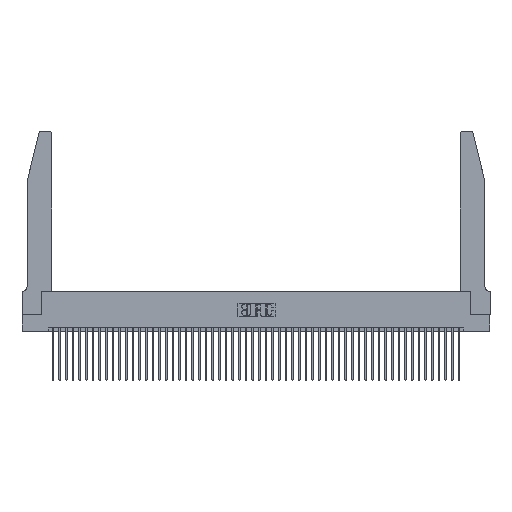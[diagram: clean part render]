
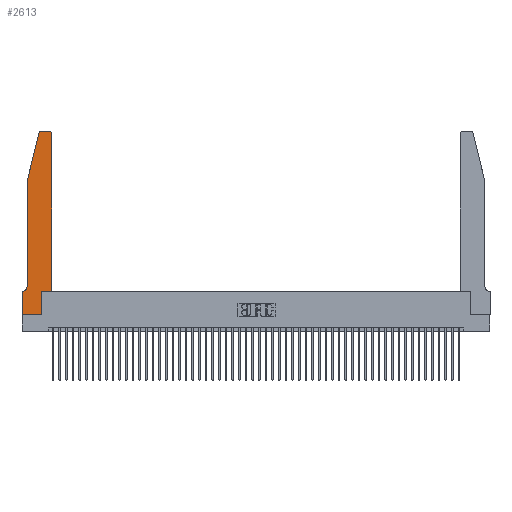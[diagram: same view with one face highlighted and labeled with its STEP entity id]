
A CAD part, top view. The second image highlights one B-rep face of the part: STEP entity #2613.
In plain terms, the highlighted planar face has unit normal (0, 0, 1).
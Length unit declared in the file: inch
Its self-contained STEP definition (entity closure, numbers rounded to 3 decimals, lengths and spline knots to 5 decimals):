
#404 = ORIENTED_EDGE ( 'NONE', *, *, #20360, .T. ) ;
#858 = CARTESIAN_POINT ( 'NONE',  ( 0., 0., 0.37 ) ) ;
#930 = CARTESIAN_POINT ( 'NONE',  ( 0.4505, 0.35, 0.37 ) ) ;
#966 = CARTESIAN_POINT ( 'NONE',  ( 0.2605, 2.75, 0.37 ) ) ;
#1242 = EDGE_CURVE ( 'NONE', #24126, #49317, #38608, .T. ) ;
#1662 = DIRECTION ( 'NONE',  ( -1., 0., 0. ) ) ;
#1768 = DIRECTION ( 'NONE',  ( 1., 0., 0. ) ) ;
#1855 = EDGE_CURVE ( 'NONE', #40231, #25761, #19600, .T. ) ;
#2353 = EDGE_CURVE ( 'NONE', #49317, #40231, #27461, .T. ) ;
#2613 = ADVANCED_FACE ( 'NONE', ( #15233 ), #11036, .T. ) ;
#3764 = CARTESIAN_POINT ( 'NONE',  ( 0.0755, 2., 0.37 ) ) ;
#3920 = CIRCLE ( 'NONE', #30477, 0.03 ) ;
#4323 = VERTEX_POINT ( 'NONE', #44053 ) ;
#4477 = VECTOR ( 'NONE', #21433, 39.37008 ) ;
#4909 = CARTESIAN_POINT ( 'NONE',  ( 0.4205, 2.72, 0.37 ) ) ;
#5491 = AXIS2_PLACEMENT_3D ( 'NONE', #30326, #15681, #43012 ) ;
#6321 = CARTESIAN_POINT ( 'NONE',  ( 0., 0., 0.37 ) ) ;
#6612 = VERTEX_POINT ( 'NONE', #23399 ) ;
#6615 = ORIENTED_EDGE ( 'NONE', *, *, #37002, .T. ) ;
#6620 = VECTOR ( 'NONE', #36160, 39.37008 ) ;
#7114 = AXIS2_PLACEMENT_3D ( 'NONE', #4909, #32318, #8887 ) ;
#7697 = CARTESIAN_POINT ( 'NONE',  ( 0.0055, 0.42, 0.37 ) ) ;
#7743 = DIRECTION ( 'NONE',  ( 0., -1., 0. ) ) ;
#8887 = DIRECTION ( 'NONE',  ( 1., 0., 0. ) ) ;
#9436 = EDGE_CURVE ( 'NONE', #43736, #24126, #42196, .T. ) ;
#11036 = PLANE ( 'NONE',  #5491 ) ;
#11334 = AXIS2_PLACEMENT_3D ( 'NONE', #7697, #35082, #11703 ) ;
#11703 = DIRECTION ( 'NONE',  ( -1., 0., 0. ) ) ;
#12312 = VERTEX_POINT ( 'NONE', #38471 ) ;
#12825 = ORIENTED_EDGE ( 'NONE', *, *, #1242, .T. ) ;
#12898 = DIRECTION ( 'NONE',  ( -1., 0., 0. ) ) ;
#13144 = EDGE_CURVE ( 'NONE', #4323, #43736, #49704, .T. ) ;
#13678 = VERTEX_POINT ( 'NONE', #22310 ) ;
#13869 = DIRECTION ( 'NONE',  ( 1., 0., 0. ) ) ;
#14236 = VECTOR ( 'NONE', #12898, 39.37008 ) ;
#14299 = VERTEX_POINT ( 'NONE', #37584 ) ;
#15233 = FACE_OUTER_BOUND ( 'NONE', #39328, .T. ) ;
#15681 = DIRECTION ( 'NONE',  ( 0., 0., 1. ) ) ;
#16694 = CIRCLE ( 'NONE', #7114, 0.03 ) ;
#17501 = CARTESIAN_POINT ( 'NONE',  ( 0.0755, 2., 0.37 ) ) ;
#18309 = ORIENTED_EDGE ( 'NONE', *, *, #13144, .T. ) ;
#18565 = VECTOR ( 'NONE', #7743, 39.37008 ) ;
#18959 = ORIENTED_EDGE ( 'NONE', *, *, #24368, .T. ) ;
#19588 = LINE ( 'NONE', #30617, #39130 ) ;
#19600 = LINE ( 'NONE', #41186, #39144 ) ;
#20360 = EDGE_CURVE ( 'NONE', #12312, #13678, #45392, .T. ) ;
#20955 = VECTOR ( 'NONE', #24671, 39.37008 ) ;
#21305 = CARTESIAN_POINT ( 'NONE',  ( 0.0755, 0.35, 0.37 ) ) ;
#21433 = DIRECTION ( 'NONE',  ( -0.239, -0.971, 0. ) ) ;
#21994 = ORIENTED_EDGE ( 'NONE', *, *, #9436, .T. ) ;
#22310 = CARTESIAN_POINT ( 'NONE',  ( 0.284, 2.75, 0.37 ) ) ;
#23399 = CARTESIAN_POINT ( 'NONE',  ( 0.25487, 2.72718, 0.37 ) ) ;
#24126 = VERTEX_POINT ( 'NONE', #45436 ) ;
#24368 = EDGE_CURVE ( 'NONE', #14299, #26873, #49420, .T. ) ;
#24671 = DIRECTION ( 'NONE',  ( 0., 1., 0. ) ) ;
#25321 = DIRECTION ( 'NONE',  ( 0., 0., 1. ) ) ;
#25738 = VERTEX_POINT ( 'NONE', #27847 ) ;
#25761 = VERTEX_POINT ( 'NONE', #47512 ) ;
#26873 = VERTEX_POINT ( 'NONE', #930 ) ;
#27461 = LINE ( 'NONE', #858, #6620 ) ;
#27847 = CARTESIAN_POINT ( 'NONE',  ( 0.4505, 2.72, 0.37 ) ) ;
#28644 = VECTOR ( 'NONE', #31398, 39.37008 ) ;
#28754 = EDGE_CURVE ( 'NONE', #25738, #12312, #16694, .T. ) ;
#29267 = CARTESIAN_POINT ( 'NONE',  ( 0., 0.35, 0.37 ) ) ;
#30247 = EDGE_CURVE ( 'NONE', #25761, #14299, #19588, .T. ) ;
#30326 = CARTESIAN_POINT ( 'NONE',  ( 0., 0.35, 0.37 ) ) ;
#30477 = AXIS2_PLACEMENT_3D ( 'NONE', #48682, #25321, #1768 ) ;
#30617 = CARTESIAN_POINT ( 'NONE',  ( 0.2865, 0.35, 0.37 ) ) ;
#31398 = DIRECTION ( 'NONE',  ( 1., 0., 0. ) ) ;
#32318 = DIRECTION ( 'NONE',  ( 0., 0., 1. ) ) ;
#32518 = LINE ( 'NONE', #44138, #20955 ) ;
#34564 = DIRECTION ( 'NONE',  ( 0., 1., 0. ) ) ;
#35082 = DIRECTION ( 'NONE',  ( 0., 0., -1. ) ) ;
#35743 = LINE ( 'NONE', #17501, #4477 ) ;
#36160 = DIRECTION ( 'NONE',  ( 0., -1., 0. ) ) ;
#37002 = EDGE_CURVE ( 'NONE', #6612, #4323, #35743, .T. ) ;
#37262 = ORIENTED_EDGE ( 'NONE', *, *, #30247, .T. ) ;
#37584 = CARTESIAN_POINT ( 'NONE',  ( 0.2865, 0.35, 0.37 ) ) ;
#38471 = CARTESIAN_POINT ( 'NONE',  ( 0.4205, 2.75, 0.37 ) ) ;
#38608 = LINE ( 'NONE', #21305, #47744 ) ;
#38744 = EDGE_CURVE ( 'NONE', #26873, #25738, #32518, .T. ) ;
#39130 = VECTOR ( 'NONE', #34564, 39.37008 ) ;
#39144 = VECTOR ( 'NONE', #13869, 39.37008 ) ;
#39328 = EDGE_LOOP ( 'NONE', ( #404, #42113, #6615, #18309, #21994, #12825, #45209, #46446, #37262, #18959, #50093, #43416 ) ) ;
#40231 = VERTEX_POINT ( 'NONE', #6321 ) ;
#41186 = CARTESIAN_POINT ( 'NONE',  ( 0., 0., 0.37 ) ) ;
#42113 = ORIENTED_EDGE ( 'NONE', *, *, #45162, .T. ) ;
#42196 = CIRCLE ( 'NONE', #11334, 0.07 ) ;
#43012 = DIRECTION ( 'NONE',  ( 1., 0., 0. ) ) ;
#43416 = ORIENTED_EDGE ( 'NONE', *, *, #28754, .T. ) ;
#43597 = CARTESIAN_POINT ( 'NONE',  ( 0.0755, 0.42, 0.37 ) ) ;
#43736 = VERTEX_POINT ( 'NONE', #43597 ) ;
#44053 = CARTESIAN_POINT ( 'NONE',  ( 0.0755, 2., 0.37 ) ) ;
#44138 = CARTESIAN_POINT ( 'NONE',  ( 0.4505, 0.35, 0.37 ) ) ;
#45162 = EDGE_CURVE ( 'NONE', #13678, #6612, #3920, .T. ) ;
#45209 = ORIENTED_EDGE ( 'NONE', *, *, #2353, .T. ) ;
#45392 = LINE ( 'NONE', #966, #14236 ) ;
#45436 = CARTESIAN_POINT ( 'NONE',  ( 0.0055, 0.35, 0.37 ) ) ;
#46446 = ORIENTED_EDGE ( 'NONE', *, *, #1855, .T. ) ;
#46962 = CARTESIAN_POINT ( 'NONE',  ( 0.4505, 0.35, 0.37 ) ) ;
#47512 = CARTESIAN_POINT ( 'NONE',  ( 0.2865, 0., 0.37 ) ) ;
#47744 = VECTOR ( 'NONE', #1662, 39.37008 ) ;
#48682 = CARTESIAN_POINT ( 'NONE',  ( 0.284, 2.72, 0.37 ) ) ;
#49317 = VERTEX_POINT ( 'NONE', #29267 ) ;
#49420 = LINE ( 'NONE', #46962, #28644 ) ;
#49704 = LINE ( 'NONE', #3764, #18565 ) ;
#50093 = ORIENTED_EDGE ( 'NONE', *, *, #38744, .T. ) ;
